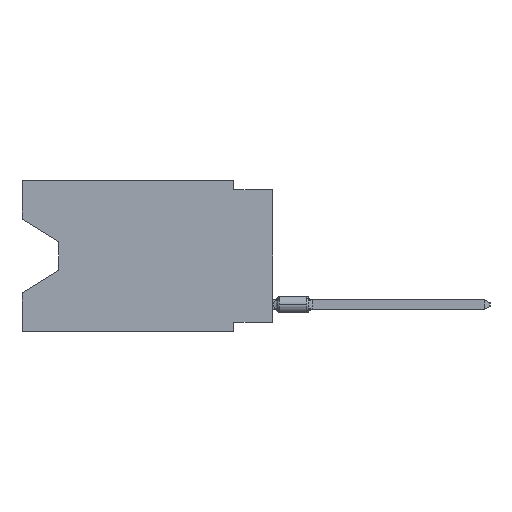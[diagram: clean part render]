
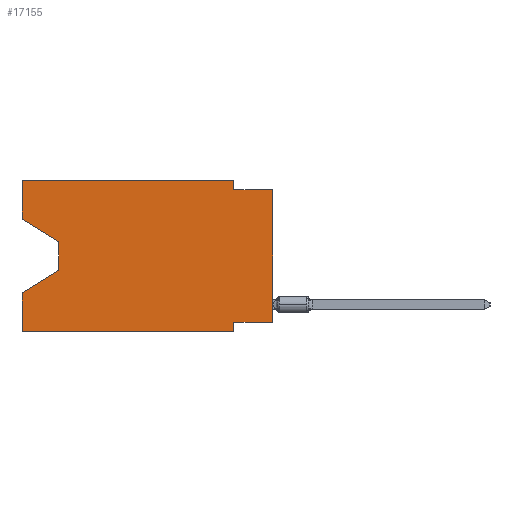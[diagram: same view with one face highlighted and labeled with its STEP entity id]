
A CAD part, left-side view. The second image highlights one B-rep face of the part: STEP entity #17155.
In plain terms, the highlighted planar face has unit normal (-1, 0, 0).
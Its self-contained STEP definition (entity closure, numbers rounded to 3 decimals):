
#294 = CARTESIAN_POINT ( 'NONE',  ( 0., 16.383, 0. ) ) ;
#529 = DIRECTION ( 'NONE',  ( 0., -1., 0. ) ) ;
#1570 = ORIENTED_EDGE ( 'NONE', *, *, #16788, .T. ) ;
#1641 = CARTESIAN_POINT ( 'NONE',  ( 0., 2.54, -0.635 ) ) ;
#1808 = CARTESIAN_POINT ( 'NONE',  ( 0., 16.383, -2.546 ) ) ;
#2499 = ORIENTED_EDGE ( 'NONE', *, *, #13835, .T. ) ;
#2570 = ORIENTED_EDGE ( 'NONE', *, *, #29485, .T. ) ;
#3163 = LINE ( 'NONE', #7065, #10955 ) ;
#3217 = ORIENTED_EDGE ( 'NONE', *, *, #16791, .F. ) ;
#3722 = EDGE_CURVE ( 'NONE', #33387, #37849, #37478, .T. ) ;
#3823 = DIRECTION ( 'NONE',  ( 0., 0.855, -0.519 ) ) ;
#4497 = EDGE_CURVE ( 'NONE', #30576, #19760, #26097, .T. ) ;
#5009 = CARTESIAN_POINT ( 'NONE',  ( 0., 16.383, 0. ) ) ;
#6463 = CARTESIAN_POINT ( 'NONE',  ( 0., 0., 0. ) ) ;
#6947 = ORIENTED_EDGE ( 'NONE', *, *, #4497, .F. ) ;
#7026 = DIRECTION ( 'NONE',  ( 0., 0., -1. ) ) ;
#7065 = CARTESIAN_POINT ( 'NONE',  ( 0., 16.383, -9.906 ) ) ;
#7363 = EDGE_CURVE ( 'NONE', #18922, #21434, #35006, .T. ) ;
#7781 = VERTEX_POINT ( 'NONE', #19688 ) ;
#7953 = VECTOR ( 'NONE', #38591, 1000. ) ;
#8237 = CARTESIAN_POINT ( 'NONE',  ( 0., 2.54, 0. ) ) ;
#9082 = DIRECTION ( 'NONE',  ( 0., 0., 1. ) ) ;
#10148 = CARTESIAN_POINT ( 'NONE',  ( 0., 16.383, 0. ) ) ;
#10305 = ORIENTED_EDGE ( 'NONE', *, *, #36967, .T. ) ;
#10335 = CARTESIAN_POINT ( 'NONE',  ( 0., 13.97, -5.893 ) ) ;
#10688 = EDGE_CURVE ( 'NONE', #21434, #21385, #41168, .T. ) ;
#10755 = LINE ( 'NONE', #37241, #39450 ) ;
#10955 = VECTOR ( 'NONE', #529, 1000. ) ;
#11060 = VECTOR ( 'NONE', #27483, 1000. ) ;
#11127 = VECTOR ( 'NONE', #33840, 1000. ) ;
#12425 = DIRECTION ( 'NONE',  ( 0., 1., 0. ) ) ;
#13548 = DIRECTION ( 'NONE',  ( 0., 0., 1. ) ) ;
#13835 = EDGE_CURVE ( 'NONE', #30576, #21385, #36216, .T. ) ;
#15895 = CARTESIAN_POINT ( 'NONE',  ( 0., 0., -9.271 ) ) ;
#16788 = EDGE_CURVE ( 'NONE', #32740, #7781, #30509, .T. ) ;
#16791 = EDGE_CURVE ( 'NONE', #19760, #27017, #10755, .T. ) ;
#17132 = CARTESIAN_POINT ( 'NONE',  ( 0., 16.383, 0. ) ) ;
#17155 = ADVANCED_FACE ( 'NONE', ( #40018 ), #23300, .F. ) ;
#18484 = VERTEX_POINT ( 'NONE', #25197 ) ;
#18888 = CARTESIAN_POINT ( 'NONE',  ( 0., 13.97, -5.893 ) ) ;
#18922 = VERTEX_POINT ( 'NONE', #8237 ) ;
#18973 = ORIENTED_EDGE ( 'NONE', *, *, #20559, .F. ) ;
#19144 = CARTESIAN_POINT ( 'NONE',  ( 0., 2.54, 0. ) ) ;
#19688 = CARTESIAN_POINT ( 'NONE',  ( 0., 16.383, -7.36 ) ) ;
#19760 = VERTEX_POINT ( 'NONE', #25202 ) ;
#19764 = CARTESIAN_POINT ( 'NONE',  ( 0., 2.54, -9.906 ) ) ;
#20475 = CARTESIAN_POINT ( 'NONE',  ( 0., 16.383, 0. ) ) ;
#20559 = EDGE_CURVE ( 'NONE', #40453, #7781, #30050, .T. ) ;
#20976 = CARTESIAN_POINT ( 'NONE',  ( 0., 0., -0.635 ) ) ;
#21385 = VERTEX_POINT ( 'NONE', #20976 ) ;
#21434 = VERTEX_POINT ( 'NONE', #1641 ) ;
#21734 = DIRECTION ( 'NONE',  ( 0., -0.855, -0.519 ) ) ;
#23300 = PLANE ( 'NONE',  #27706 ) ;
#23618 = VECTOR ( 'NONE', #12425, 1000. ) ;
#24652 = CARTESIAN_POINT ( 'NONE',  ( 0., 0., -0.635 ) ) ;
#25183 = EDGE_CURVE ( 'NONE', #33387, #18484, #34130, .T. ) ;
#25197 = CARTESIAN_POINT ( 'NONE',  ( 0., 13.97, -4.013 ) ) ;
#25202 = CARTESIAN_POINT ( 'NONE',  ( 0., 2.54, -9.271 ) ) ;
#26015 = CARTESIAN_POINT ( 'NONE',  ( 0., 16.383, -9.906 ) ) ;
#26097 = LINE ( 'NONE', #15895, #23618 ) ;
#26836 = ORIENTED_EDGE ( 'NONE', *, *, #7363, .F. ) ;
#27017 = VERTEX_POINT ( 'NONE', #19764 ) ;
#27109 = VECTOR ( 'NONE', #31181, 1000. ) ;
#27237 = VECTOR ( 'NONE', #13548, 1000. ) ;
#27243 = DIRECTION ( 'NONE',  ( 0., 0., -1. ) ) ;
#27483 = DIRECTION ( 'NONE',  ( 0., 0., 1. ) ) ;
#27706 = AXIS2_PLACEMENT_3D ( 'NONE', #20475, #36557, #7026 ) ;
#28686 = VECTOR ( 'NONE', #9082, 1000. ) ;
#29128 = DIRECTION ( 'NONE',  ( 0., 0., -1. ) ) ;
#29485 = EDGE_CURVE ( 'NONE', #40453, #27017, #3163, .T. ) ;
#29948 = CARTESIAN_POINT ( 'NONE',  ( 0., 0., -9.271 ) ) ;
#30050 = LINE ( 'NONE', #294, #27237 ) ;
#30437 = VECTOR ( 'NONE', #3823, 1000. ) ;
#30509 = LINE ( 'NONE', #10335, #30437 ) ;
#30576 = VERTEX_POINT ( 'NONE', #29948 ) ;
#30589 = LINE ( 'NONE', #17132, #11127 ) ;
#31064 = LINE ( 'NONE', #37362, #7953 ) ;
#31181 = DIRECTION ( 'NONE',  ( 0., -1., 0. ) ) ;
#31302 = CARTESIAN_POINT ( 'NONE',  ( 0., 16.383, -2.546 ) ) ;
#31796 = ORIENTED_EDGE ( 'NONE', *, *, #10688, .F. ) ;
#32740 = VERTEX_POINT ( 'NONE', #18888 ) ;
#32918 = EDGE_CURVE ( 'NONE', #37849, #18922, #30589, .T. ) ;
#33387 = VERTEX_POINT ( 'NONE', #1808 ) ;
#33840 = DIRECTION ( 'NONE',  ( 0., -1., 0. ) ) ;
#34130 = LINE ( 'NONE', #31302, #36461 ) ;
#35006 = LINE ( 'NONE', #19144, #38401 ) ;
#36216 = LINE ( 'NONE', #6463, #28686 ) ;
#36461 = VECTOR ( 'NONE', #21734, 1000. ) ;
#36557 = DIRECTION ( 'NONE',  ( 1., 0., 0. ) ) ;
#36967 = EDGE_CURVE ( 'NONE', #18484, #32740, #31064, .T. ) ;
#37241 = CARTESIAN_POINT ( 'NONE',  ( 0., 2.54, -9.906 ) ) ;
#37362 = CARTESIAN_POINT ( 'NONE',  ( 0., 13.97, -4.013 ) ) ;
#37478 = LINE ( 'NONE', #10148, #11060 ) ;
#37849 = VERTEX_POINT ( 'NONE', #5009 ) ;
#37953 = ORIENTED_EDGE ( 'NONE', *, *, #25183, .T. ) ;
#38401 = VECTOR ( 'NONE', #29128, 1000. ) ;
#38574 = ORIENTED_EDGE ( 'NONE', *, *, #32918, .F. ) ;
#38591 = DIRECTION ( 'NONE',  ( 0., 0., -1. ) ) ;
#39038 = ORIENTED_EDGE ( 'NONE', *, *, #3722, .F. ) ;
#39450 = VECTOR ( 'NONE', #27243, 1000. ) ;
#40018 = FACE_OUTER_BOUND ( 'NONE', #40064, .T. ) ;
#40064 = EDGE_LOOP ( 'NONE', ( #37953, #10305, #1570, #18973, #2570, #3217, #6947, #2499, #31796, #26836, #38574, #39038 ) ) ;
#40453 = VERTEX_POINT ( 'NONE', #26015 ) ;
#41168 = LINE ( 'NONE', #24652, #27109 ) ;
